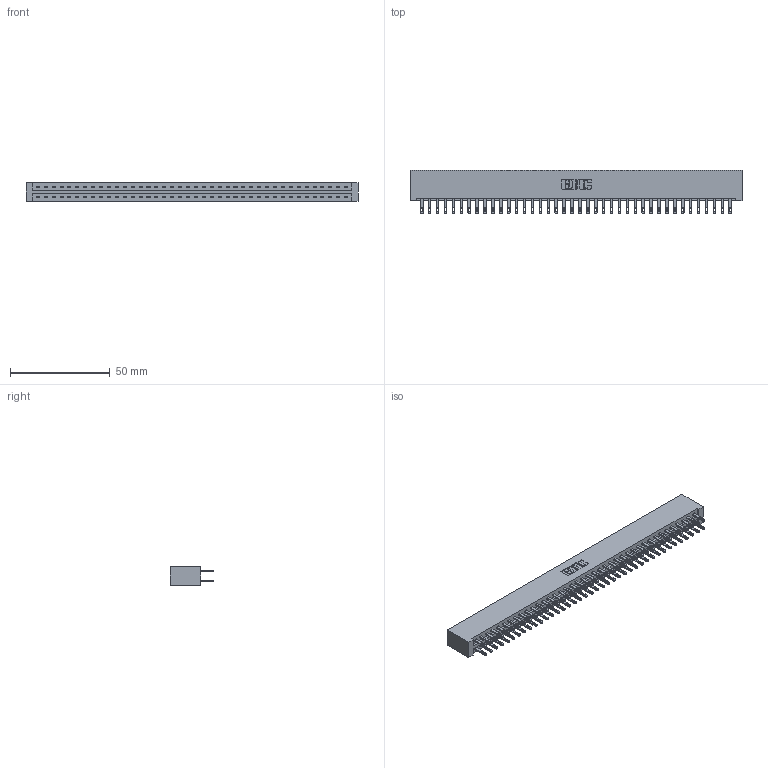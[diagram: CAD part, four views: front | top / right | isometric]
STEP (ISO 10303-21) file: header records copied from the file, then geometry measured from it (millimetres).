
FILE_DESCRIPTION (( 'STEP AP203' ), '1' );
FILE_NAME ('337-080-500-201.STEP', '2019-10-10T11:51:25', ( '' ), ( '' ), 'SwSTEP 2.0', 'SolidWorks 2016', '' );
FILE_SCHEMA (( 'CONFIG_CONTROL_DESIGN' ));
Length unit declared in the file: inch
Products named in the file (3): 337 Part_No Mounting Lugs; 337-080-500-201; 345-292-001_345-293-100
Assembly tree (81 placements, depth 2):
  337-080-500-201
    337 Part_No Mounting Lugs
    345-292-001_345-293-100  x80
Bounding box: 166.37 x 21.85 x 9.4 mm (x, y, z)
Volume: 18512 mm3; surface area: 21852.2 mm2
Topology: 81 solids, 81 shells, 4106 faces, 12527 edges, 8350 vertices
Faces by surface type: plane 2626, cylinder 1480
Entity records: 30925 total; most frequent: CARTESIAN_POINT 5210, ORIENTED_EDGE 5146, DIRECTION 4429, EDGE_CURVE 2573, LINE 2449, VECTOR 2449, VERTEX_POINT 1714, AXIS2_PLACEMENT_3D 990
